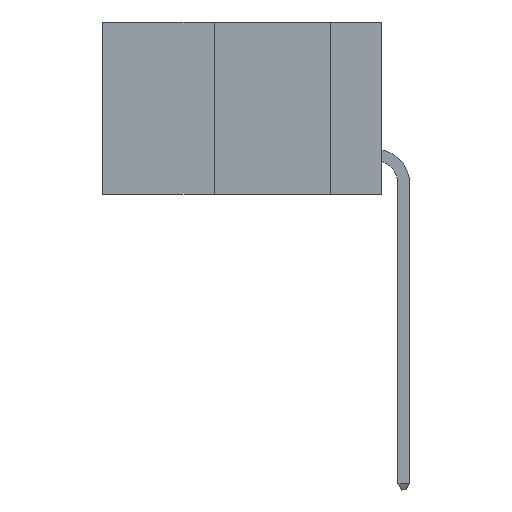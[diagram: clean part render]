
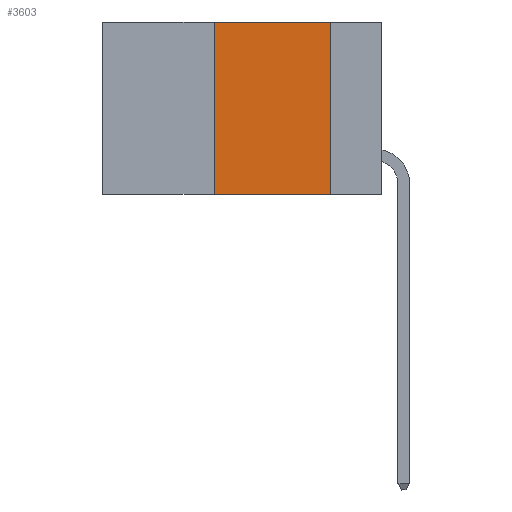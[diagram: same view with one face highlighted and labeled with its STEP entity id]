
A CAD part, left-side view. The second image highlights one B-rep face of the part: STEP entity #3603.
In plain terms, the highlighted planar face has unit normal (-1, 0, 0).
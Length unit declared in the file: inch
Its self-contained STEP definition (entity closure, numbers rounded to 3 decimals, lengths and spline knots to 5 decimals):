
#171 = DIRECTION ( 'NONE',  ( 0., -1., 0. ) ) ;
#282 = CARTESIAN_POINT ( 'NONE',  ( 0., 0.11, 0. ) ) ;
#466 = EDGE_CURVE ( 'NONE', #10109, #5144, #2858, .T. ) ;
#595 = FACE_OUTER_BOUND ( 'NONE', #11082, .T. ) ;
#1201 = DIRECTION ( 'NONE',  ( 0., 0., -1. ) ) ;
#1321 = PLANE ( 'NONE',  #8575 ) ;
#2135 = DIRECTION ( 'NONE',  ( 0., 0., -1. ) ) ;
#2720 = EDGE_CURVE ( 'NONE', #6343, #10343, #5701, .T. ) ;
#2858 = LINE ( 'NONE', #3699, #7799 ) ;
#3483 = LINE ( 'NONE', #8497, #8019 ) ;
#3603 = ADVANCED_FACE ( 'NONE', ( #595 ), #1321, .F. ) ;
#3699 = CARTESIAN_POINT ( 'NONE',  ( 0., 0.6, 0. ) ) ;
#4868 = ORIENTED_EDGE ( 'NONE', *, *, #8970, .F. ) ;
#5144 = VERTEX_POINT ( 'NONE', #282 ) ;
#5522 = LINE ( 'NONE', #8602, #9741 ) ;
#5548 = CARTESIAN_POINT ( 'NONE',  ( 0., 0.36, 0. ) ) ;
#5701 = LINE ( 'NONE', #6821, #6309 ) ;
#5892 = ORIENTED_EDGE ( 'NONE', *, *, #9714, .F. ) ;
#6065 = DIRECTION ( 'NONE',  ( 0., -1., 0. ) ) ;
#6309 = VECTOR ( 'NONE', #171, 39.37008 ) ;
#6343 = VERTEX_POINT ( 'NONE', #6701 ) ;
#6701 = CARTESIAN_POINT ( 'NONE',  ( 0., 0.36, -0.37 ) ) ;
#6821 = CARTESIAN_POINT ( 'NONE',  ( 0., 0.6, -0.37 ) ) ;
#7555 = CARTESIAN_POINT ( 'NONE',  ( 0., 0.11, -0.37 ) ) ;
#7748 = CARTESIAN_POINT ( 'NONE',  ( 0., 0.6, 0. ) ) ;
#7799 = VECTOR ( 'NONE', #6065, 39.37008 ) ;
#7828 = DIRECTION ( 'NONE',  ( 1., 0., 0. ) ) ;
#8019 = VECTOR ( 'NONE', #11248, 39.37008 ) ;
#8497 = CARTESIAN_POINT ( 'NONE',  ( 0., 0.36, 0. ) ) ;
#8575 = AXIS2_PLACEMENT_3D ( 'NONE', #7748, #7828, #2135 ) ;
#8602 = CARTESIAN_POINT ( 'NONE',  ( 0., 0.11, 0. ) ) ;
#8970 = EDGE_CURVE ( 'NONE', #6343, #10109, #3483, .T. ) ;
#9714 = EDGE_CURVE ( 'NONE', #5144, #10343, #5522, .T. ) ;
#9741 = VECTOR ( 'NONE', #1201, 39.37008 ) ;
#10109 = VERTEX_POINT ( 'NONE', #5548 ) ;
#10343 = VERTEX_POINT ( 'NONE', #7555 ) ;
#11034 = ORIENTED_EDGE ( 'NONE', *, *, #466, .F. ) ;
#11082 = EDGE_LOOP ( 'NONE', ( #5892, #11034, #4868, #11106 ) ) ;
#11106 = ORIENTED_EDGE ( 'NONE', *, *, #2720, .T. ) ;
#11248 = DIRECTION ( 'NONE',  ( 0., 0., 1. ) ) ;
